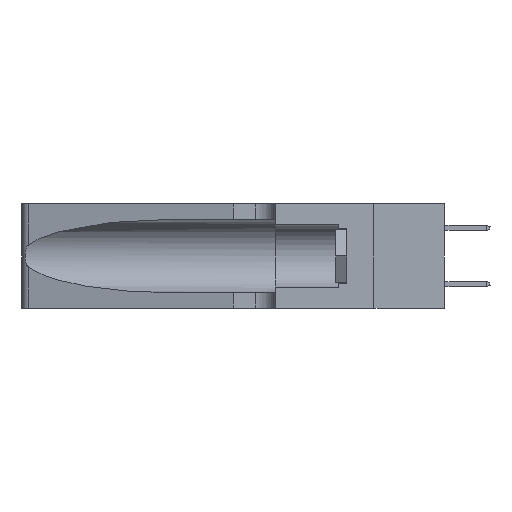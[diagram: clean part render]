
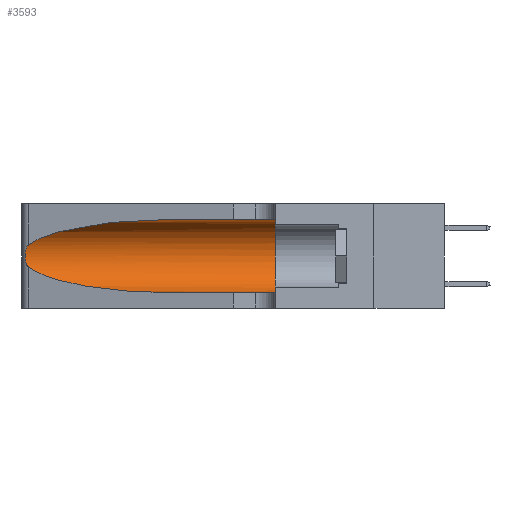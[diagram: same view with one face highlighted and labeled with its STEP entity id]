
A CAD part, left-side view. The second image highlights one B-rep face of the part: STEP entity #3593.
In plain terms, the highlighted cylindrical face has radius 3.308 mm (diameter 6.617 mm), a partial arc.
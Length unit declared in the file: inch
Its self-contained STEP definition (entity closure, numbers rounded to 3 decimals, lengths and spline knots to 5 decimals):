
#27 = CARTESIAN_POINT ( 'NONE',  ( 0.1305, 0.35, 0.185 ) ) ;
#1093 = ORIENTED_EDGE ( 'NONE', *, *, #17574, .F. ) ;
#1156 = EDGE_LOOP ( 'NONE', ( #28761, #21807, #2742, #25230, #1093, #17047 ) ) ;
#2581 = CARTESIAN_POINT ( 'NONE',  ( 0.25487, 1.22718, 0.22369 ) ) ;
#2713 = CARTESIAN_POINT ( 'NONE',  ( 0.25555, 1.22993, 0.14849 ) ) ;
#2742 = ORIENTED_EDGE ( 'NONE', *, *, #8621, .T. ) ;
#3045 = VECTOR ( 'NONE', #23397, 39.37008 ) ;
#3091 = DIRECTION ( 'NONE',  ( 0., 0., 1. ) ) ;
#3207 = CARTESIAN_POINT ( 'NONE',  ( 0.1305, 0.72297, 0.31525 ) ) ;
#3563 = DIRECTION ( 'NONE',  ( 0., -1., 0. ) ) ;
#3593 = ADVANCED_FACE ( 'NONE', ( #32846 ), #9157, .F. ) ;
#3619 = VERTEX_POINT ( 'NONE', #12491 ) ;
#5189 = CARTESIAN_POINT ( 'NONE',  ( 0.2373, 1.15595, 0.08982 ) ) ;
#5565 = CARTESIAN_POINT ( 'NONE',  ( 0.25555, 1.22994, 0.2215 ) ) ;
#5600 = CARTESIAN_POINT ( 'NONE',  ( 0.1305, 1.61858, 0.31525 ) ) ;
#5659 = EDGE_CURVE ( 'NONE', #29538, #31817, #19043, .T. ) ;
#6162 = CARTESIAN_POINT ( 'NONE',  ( 0.18966, 0.96281, 0.31525 ) ) ;
#6425 = CARTESIAN_POINT ( 'NONE',  ( 0.25487, 1.22718, 0.14631 ) ) ;
#6713 = AXIS2_PLACEMENT_3D ( 'NONE', #27, #20889, #3091 ) ;
#7002 = EDGE_CURVE ( 'NONE', #36864, #21913, #11830, .T. ) ;
#7335 = VERTEX_POINT ( 'NONE', #36854 ) ;
#7590 = EDGE_CURVE ( 'NONE', #36864, #29538, #25166, .T. ) ;
#8535 = CARTESIAN_POINT ( 'NONE',  ( 0.25787, 1.23484, 0.2124 ) ) ;
#8621 = EDGE_CURVE ( 'NONE', #31817, #3619, #11310, .T. ) ;
#9157 = CYLINDRICAL_SURFACE ( 'NONE', #34559, 0.13025 ) ;
#11151 = CARTESIAN_POINT ( 'NONE',  ( 0.1305, 0.72297, 0.05475 ) ) ;
#11310 =( BOUNDED_CURVE ( )  B_SPLINE_CURVE ( 3, ( #37757, #5189, #28957, #11151 ),
 .UNSPECIFIED., .F., .T. ) 
 B_SPLINE_CURVE_WITH_KNOTS ( ( 4, 4 ),
 ( 3.44316, 4.71239 ),
 .UNSPECIFIED. ) 
 CURVE ( )  GEOMETRIC_REPRESENTATION_ITEM ( )  RATIONAL_B_SPLINE_CURVE ( ( 1., 0.87, 0.87, 1. ) ) 
 REPRESENTATION_ITEM ( '' )  );
#11520 = CARTESIAN_POINT ( 'NONE',  ( 0.26018, 1.23835, 0.19895 ) ) ;
#11830 = LINE ( 'NONE', #5600, #3045 ) ;
#12491 = CARTESIAN_POINT ( 'NONE',  ( 0.1305, 0.72297, 0.05475 ) ) ;
#12864 = CARTESIAN_POINT ( 'NONE',  ( 0.1305, 1.61858, 0.05475 ) ) ;
#13307 = LINE ( 'NONE', #12864, #28201 ) ;
#14507 = CARTESIAN_POINT ( 'NONE',  ( 0.26075, 1.23896, 0.178 ) ) ;
#15122 = CARTESIAN_POINT ( 'NONE',  ( 0.2373, 1.15595, 0.28018 ) ) ;
#17047 = ORIENTED_EDGE ( 'NONE', *, *, #7002, .F. ) ;
#17533 = CARTESIAN_POINT ( 'NONE',  ( 0.25856, 1.23593, 0.16098 ) ) ;
#17574 = EDGE_CURVE ( 'NONE', #21913, #7335, #30263, .T. ) ;
#19043 = B_SPLINE_CURVE_WITH_KNOTS ( 'NONE', 3,
 ( #2581, #5565, #23356, #8535, #29322, #11520, #32308, #14507, #35289, #17533, #38232, #20524, #2713, #23494 ),
 .UNSPECIFIED., .F., .F.,
 ( 4, 2, 2, 2, 2, 2, 4 ),
 ( 0., 0.00027, 0.00053, 0.00107, 0.0016, 0.00187, 0.00214 ),
 .UNSPECIFIED. ) ;
#20524 = CARTESIAN_POINT ( 'NONE',  ( 0.25639, 1.23186, 0.15144 ) ) ;
#20889 = DIRECTION ( 'NONE',  ( 0., 1., 0. ) ) ;
#21373 = CARTESIAN_POINT ( 'NONE',  ( 0.1305, 1.61858, 0.185 ) ) ;
#21807 = ORIENTED_EDGE ( 'NONE', *, *, #5659, .T. ) ;
#21913 = VERTEX_POINT ( 'NONE', #22931 ) ;
#22931 = CARTESIAN_POINT ( 'NONE',  ( 0.1305, 0.35, 0.31525 ) ) ;
#23356 = CARTESIAN_POINT ( 'NONE',  ( 0.25639, 1.23184, 0.21858 ) ) ;
#23397 = DIRECTION ( 'NONE',  ( 0., -1., 0. ) ) ;
#23494 = CARTESIAN_POINT ( 'NONE',  ( 0.25487, 1.22718, 0.14631 ) ) ;
#23647 = EDGE_CURVE ( 'NONE', #3619, #7335, #13307, .T. ) ;
#24346 = DIRECTION ( 'NONE',  ( 0., 0., -1. ) ) ;
#25166 =( BOUNDED_CURVE ( )  B_SPLINE_CURVE ( 3, ( #3207, #6162, #15122, #35884 ),
 .UNSPECIFIED., .F., .T. ) 
 B_SPLINE_CURVE_WITH_KNOTS ( ( 4, 4 ),
 ( 1.5708, 2.84003 ),
 .UNSPECIFIED. ) 
 CURVE ( )  GEOMETRIC_REPRESENTATION_ITEM ( )  RATIONAL_B_SPLINE_CURVE ( ( 1., 0.87, 0.87, 1. ) ) 
 REPRESENTATION_ITEM ( '' )  );
#25230 = ORIENTED_EDGE ( 'NONE', *, *, #23647, .T. ) ;
#28201 = VECTOR ( 'NONE', #36634, 39.37008 ) ;
#28761 = ORIENTED_EDGE ( 'NONE', *, *, #7590, .T. ) ;
#28957 = CARTESIAN_POINT ( 'NONE',  ( 0.18966, 0.96281, 0.05475 ) ) ;
#29322 = CARTESIAN_POINT ( 'NONE',  ( 0.25854, 1.2359, 0.20912 ) ) ;
#29538 = VERTEX_POINT ( 'NONE', #29557 ) ;
#29557 = CARTESIAN_POINT ( 'NONE',  ( 0.25487, 1.22718, 0.22369 ) ) ;
#30263 = CIRCLE ( 'NONE', #6713, 0.13025 ) ;
#31817 = VERTEX_POINT ( 'NONE', #6425 ) ;
#32308 = CARTESIAN_POINT ( 'NONE',  ( 0.26075, 1.23896, 0.19203 ) ) ;
#32846 = FACE_OUTER_BOUND ( 'NONE', #1156, .T. ) ;
#34559 = AXIS2_PLACEMENT_3D ( 'NONE', #21373, #3563, #24346 ) ;
#35289 = CARTESIAN_POINT ( 'NONE',  ( 0.26017, 1.23833, 0.17102 ) ) ;
#35884 = CARTESIAN_POINT ( 'NONE',  ( 0.25487, 1.22718, 0.22369 ) ) ;
#36190 = CARTESIAN_POINT ( 'NONE',  ( 0.1305, 0.72297, 0.31525 ) ) ;
#36634 = DIRECTION ( 'NONE',  ( 0., -1., 0. ) ) ;
#36854 = CARTESIAN_POINT ( 'NONE',  ( 0.1305, 0.35, 0.05475 ) ) ;
#36864 = VERTEX_POINT ( 'NONE', #36190 ) ;
#37757 = CARTESIAN_POINT ( 'NONE',  ( 0.25487, 1.22718, 0.14631 ) ) ;
#38232 = CARTESIAN_POINT ( 'NONE',  ( 0.25789, 1.23486, 0.15765 ) ) ;
